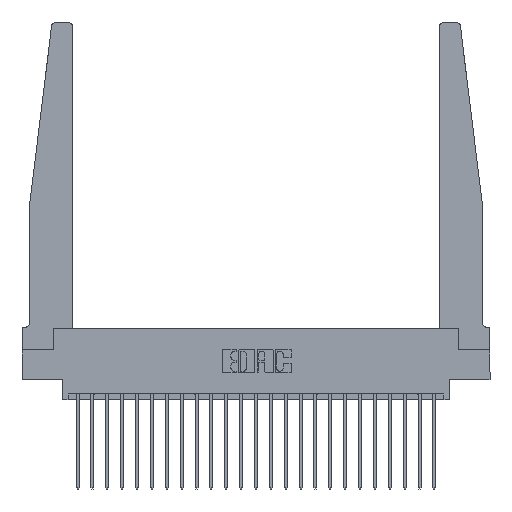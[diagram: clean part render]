
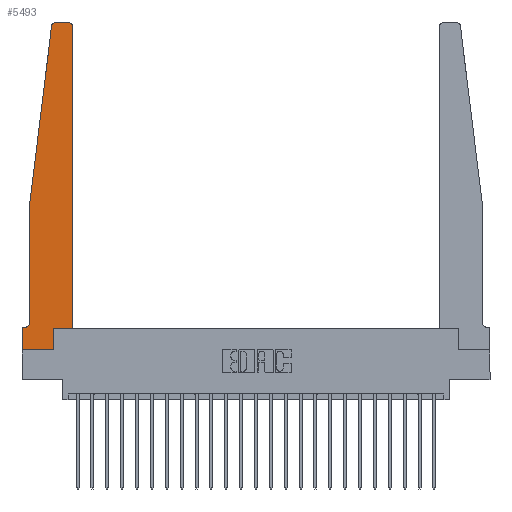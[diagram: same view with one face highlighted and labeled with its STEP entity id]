
A CAD part, top view. The second image highlights one B-rep face of the part: STEP entity #5493.
In plain terms, the highlighted planar face has unit normal (0, 0, 1).
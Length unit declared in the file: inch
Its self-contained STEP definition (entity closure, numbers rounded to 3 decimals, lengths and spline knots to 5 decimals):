
#1209 = CIRCLE ( 'NONE', #19799, 0.03 ) ;
#1280 = LINE ( 'NONE', #16089, #16244 ) ;
#1428 = DIRECTION ( 'NONE',  ( 1., 0., 0. ) ) ;
#1475 = VERTEX_POINT ( 'NONE', #4006 ) ;
#1893 = VERTEX_POINT ( 'NONE', #16958 ) ;
#2322 = EDGE_CURVE ( 'NONE', #1475, #8422, #7004, .T. ) ;
#2567 = EDGE_CURVE ( 'NONE', #4337, #23877, #2679, .T. ) ;
#2679 = CIRCLE ( 'NONE', #16245, 0.05 ) ;
#2715 = VECTOR ( 'NONE', #5414, 39.37008 ) ;
#2857 = CARTESIAN_POINT ( 'NONE',  ( 0.015, 0.1875, 0.37 ) ) ;
#2989 = LINE ( 'NONE', #21546, #6890 ) ;
#3052 = LINE ( 'NONE', #15676, #11242 ) ;
#3380 = VECTOR ( 'NONE', #5050, 39.37008 ) ;
#3398 = VERTEX_POINT ( 'NONE', #16963 ) ;
#3498 = DIRECTION ( 'NONE',  ( 1., 0., 0. ) ) ;
#3876 = CARTESIAN_POINT ( 'NONE',  ( 0.065, 1.25, 0.37 ) ) ;
#4006 = CARTESIAN_POINT ( 'NONE',  ( 0.24675, 2.72367, 0.37 ) ) ;
#4333 = LINE ( 'NONE', #23132, #8111 ) ;
#4337 = VERTEX_POINT ( 'NONE', #17630 ) ;
#5050 = DIRECTION ( 'NONE',  ( 0., 1., 0. ) ) ;
#5110 = DIRECTION ( 'NONE',  ( -1., 0., 0. ) ) ;
#5414 = DIRECTION ( 'NONE',  ( -1., 0., 0. ) ) ;
#5457 = ORIENTED_EDGE ( 'NONE', *, *, #2322, .T. ) ;
#5493 = ADVANCED_FACE ( 'NONE', ( #23853 ), #22037, .T. ) ;
#5815 = VECTOR ( 'NONE', #12565, 39.37008 ) ;
#6253 = CARTESIAN_POINT ( 'NONE',  ( 0.27653, 2.75, 0.37 ) ) ;
#6890 = VECTOR ( 'NONE', #14035, 39.37008 ) ;
#6926 = VERTEX_POINT ( 'NONE', #6253 ) ;
#7004 = LINE ( 'NONE', #14396, #5815 ) ;
#7250 = CARTESIAN_POINT ( 'NONE',  ( 0., 0.1875, 0.37 ) ) ;
#7544 = EDGE_LOOP ( 'NONE', ( #15956, #10798, #5457, #8426, #13714, #15443, #9101, #9525, #12998, #23189, #21256, #16509 ) ) ;
#8111 = VECTOR ( 'NONE', #12095, 39.37008 ) ;
#8117 = VERTEX_POINT ( 'NONE', #8990 ) ;
#8119 = LINE ( 'NONE', #15043, #23849 ) ;
#8191 = EDGE_CURVE ( 'NONE', #19653, #6926, #8119, .T. ) ;
#8422 = VERTEX_POINT ( 'NONE', #17583 ) ;
#8426 = ORIENTED_EDGE ( 'NONE', *, *, #19296, .T. ) ;
#8990 = CARTESIAN_POINT ( 'NONE',  ( 0.2605, 0., 0.37 ) ) ;
#9076 = LINE ( 'NONE', #10535, #2715 ) ;
#9101 = ORIENTED_EDGE ( 'NONE', *, *, #14045, .T. ) ;
#9525 = ORIENTED_EDGE ( 'NONE', *, *, #12953, .T. ) ;
#9616 = CIRCLE ( 'NONE', #10023, 0.03 ) ;
#10023 = AXIS2_PLACEMENT_3D ( 'NONE', #16726, #12956, #3498 ) ;
#10157 = CARTESIAN_POINT ( 'NONE',  ( 0.2605, 0.18, 0.37 ) ) ;
#10223 = DIRECTION ( 'NONE',  ( 0., 1., 0. ) ) ;
#10521 = EDGE_CURVE ( 'NONE', #3398, #16836, #2989, .T. ) ;
#10530 = EDGE_CURVE ( 'NONE', #8117, #3398, #23479, .T. ) ;
#10535 = CARTESIAN_POINT ( 'NONE',  ( 0.065, 0.1875, 0.37 ) ) ;
#10798 = ORIENTED_EDGE ( 'NONE', *, *, #11577, .T. ) ;
#11242 = VECTOR ( 'NONE', #10223, 39.37008 ) ;
#11518 = DIRECTION ( 'NONE',  ( -1., 0., 0. ) ) ;
#11577 = EDGE_CURVE ( 'NONE', #6926, #1475, #9616, .T. ) ;
#11830 = CARTESIAN_POINT ( 'NONE',  ( 0.425, 0.18, 0.37 ) ) ;
#12095 = DIRECTION ( 'NONE',  ( 0., -1., 0. ) ) ;
#12565 = DIRECTION ( 'NONE',  ( -0.122, -0.992, 0. ) ) ;
#12813 = DIRECTION ( 'NONE',  ( 1., 0., 0. ) ) ;
#12825 = CARTESIAN_POINT ( 'NONE',  ( 0.395, 2.75, 0.37 ) ) ;
#12914 = VECTOR ( 'NONE', #12973, 39.37008 ) ;
#12953 = EDGE_CURVE ( 'NONE', #19100, #8117, #1280, .T. ) ;
#12956 = DIRECTION ( 'NONE',  ( 0., 0., 1. ) ) ;
#12973 = DIRECTION ( 'NONE',  ( 0., -1., 0. ) ) ;
#12998 = ORIENTED_EDGE ( 'NONE', *, *, #10530, .T. ) ;
#13714 = ORIENTED_EDGE ( 'NONE', *, *, #2567, .T. ) ;
#14035 = DIRECTION ( 'NONE',  ( 1., 0., 0. ) ) ;
#14045 = EDGE_CURVE ( 'NONE', #1893, #19100, #4333, .T. ) ;
#14148 = CARTESIAN_POINT ( 'NONE',  ( 0.425, 2.72, 0.37 ) ) ;
#14334 = DIRECTION ( 'NONE',  ( 0., 0., -1. ) ) ;
#14396 = CARTESIAN_POINT ( 'NONE',  ( 0.065, 1.25, 0.37 ) ) ;
#15043 = CARTESIAN_POINT ( 'NONE',  ( 0.25, 2.75, 0.37 ) ) ;
#15089 = EDGE_CURVE ( 'NONE', #16836, #22797, #3052, .T. ) ;
#15443 = ORIENTED_EDGE ( 'NONE', *, *, #21190, .T. ) ;
#15676 = CARTESIAN_POINT ( 'NONE',  ( 0.425, 0.18, 0.37 ) ) ;
#15956 = ORIENTED_EDGE ( 'NONE', *, *, #8191, .T. ) ;
#16089 = CARTESIAN_POINT ( 'NONE',  ( 0., 0., 0.37 ) ) ;
#16244 = VECTOR ( 'NONE', #23480, 39.37008 ) ;
#16245 = AXIS2_PLACEMENT_3D ( 'NONE', #19316, #14334, #5110 ) ;
#16509 = ORIENTED_EDGE ( 'NONE', *, *, #22530, .T. ) ;
#16726 = CARTESIAN_POINT ( 'NONE',  ( 0.27653, 2.72, 0.37 ) ) ;
#16836 = VERTEX_POINT ( 'NONE', #11830 ) ;
#16958 = CARTESIAN_POINT ( 'NONE',  ( 0., 0.1875, 0.37 ) ) ;
#16963 = CARTESIAN_POINT ( 'NONE',  ( 0.2605, 0.18, 0.37 ) ) ;
#17583 = CARTESIAN_POINT ( 'NONE',  ( 0.065, 1.25, 0.37 ) ) ;
#17630 = CARTESIAN_POINT ( 'NONE',  ( 0.065, 0.2375, 0.37 ) ) ;
#19100 = VERTEX_POINT ( 'NONE', #23764 ) ;
#19296 = EDGE_CURVE ( 'NONE', #8422, #4337, #23892, .T. ) ;
#19316 = CARTESIAN_POINT ( 'NONE',  ( 0.015, 0.2375, 0.37 ) ) ;
#19653 = VERTEX_POINT ( 'NONE', #12825 ) ;
#19799 = AXIS2_PLACEMENT_3D ( 'NONE', #21925, #22164, #1428 ) ;
#20729 = AXIS2_PLACEMENT_3D ( 'NONE', #7250, #22510, #12813 ) ;
#21190 = EDGE_CURVE ( 'NONE', #23877, #1893, #9076, .T. ) ;
#21256 = ORIENTED_EDGE ( 'NONE', *, *, #15089, .T. ) ;
#21546 = CARTESIAN_POINT ( 'NONE',  ( 0.425, 0.18, 0.37 ) ) ;
#21925 = CARTESIAN_POINT ( 'NONE',  ( 0.395, 2.72, 0.37 ) ) ;
#22037 = PLANE ( 'NONE',  #20729 ) ;
#22164 = DIRECTION ( 'NONE',  ( 0., 0., 1. ) ) ;
#22510 = DIRECTION ( 'NONE',  ( 0., 0., 1. ) ) ;
#22530 = EDGE_CURVE ( 'NONE', #22797, #19653, #1209, .T. ) ;
#22797 = VERTEX_POINT ( 'NONE', #14148 ) ;
#23132 = CARTESIAN_POINT ( 'NONE',  ( 0., 0., 0.37 ) ) ;
#23189 = ORIENTED_EDGE ( 'NONE', *, *, #10521, .T. ) ;
#23479 = LINE ( 'NONE', #10157, #3380 ) ;
#23480 = DIRECTION ( 'NONE',  ( 1., 0., 0. ) ) ;
#23764 = CARTESIAN_POINT ( 'NONE',  ( 0., 0., 0.37 ) ) ;
#23849 = VECTOR ( 'NONE', #11518, 39.37008 ) ;
#23853 = FACE_OUTER_BOUND ( 'NONE', #7544, .T. ) ;
#23877 = VERTEX_POINT ( 'NONE', #2857 ) ;
#23892 = LINE ( 'NONE', #3876, #12914 ) ;
